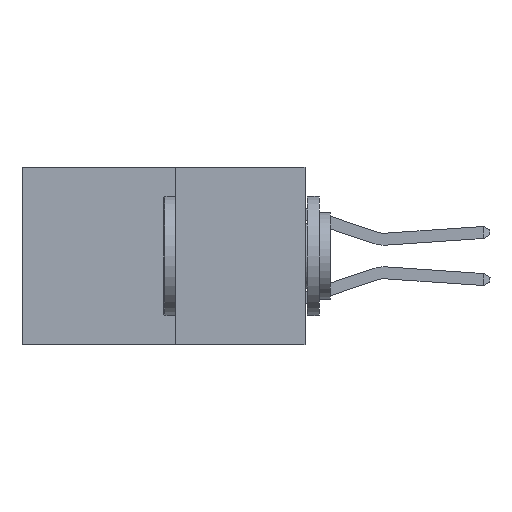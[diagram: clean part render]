
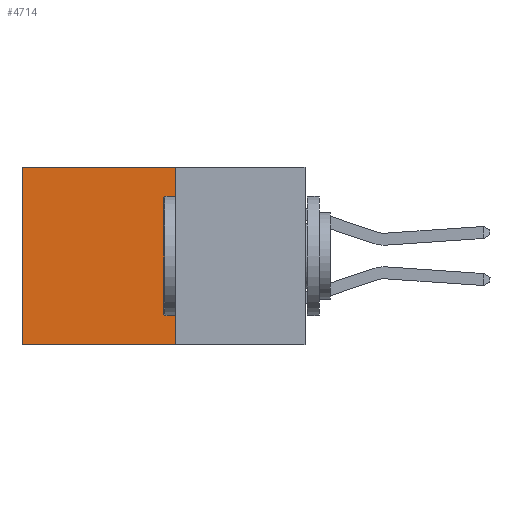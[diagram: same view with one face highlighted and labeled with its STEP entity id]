
A CAD part, left-side view. The second image highlights one B-rep face of the part: STEP entity #4714.
In plain terms, the highlighted planar face has unit normal (-1, 0, 0).
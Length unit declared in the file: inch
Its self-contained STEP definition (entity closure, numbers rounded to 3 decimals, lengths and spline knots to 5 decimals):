
#1151 = VERTEX_POINT ( 'NONE', #15714 ) ;
#1609 = EDGE_CURVE ( 'NONE', #25152, #21305, #25928, .T. ) ;
#1952 = LINE ( 'NONE', #5061, #23638 ) ;
#2919 = EDGE_LOOP ( 'NONE', ( #13480, #12660, #11735, #12608 ) ) ;
#3179 = CARTESIAN_POINT ( 'NONE',  ( 0.277, 0.59, -0.37 ) ) ;
#3272 = VERTEX_POINT ( 'NONE', #8045 ) ;
#3639 = VECTOR ( 'NONE', #25859, 39.37008 ) ;
#4335 = PLANE ( 'NONE',  #7611 ) ;
#4714 = ADVANCED_FACE ( 'NONE', ( #8375 ), #4335, .F. ) ;
#5060 = DIRECTION ( 'NONE',  ( 0., 1., 0. ) ) ;
#5061 = CARTESIAN_POINT ( 'NONE',  ( 0.277, 0.27, -0.37 ) ) ;
#6371 = DIRECTION ( 'NONE',  ( 0., 1., 0. ) ) ;
#7062 = EDGE_CURVE ( 'NONE', #1151, #3272, #1952, .T. ) ;
#7527 = LINE ( 'NONE', #11397, #11865 ) ;
#7611 = AXIS2_PLACEMENT_3D ( 'NONE', #21199, #8630, #23264 ) ;
#8045 = CARTESIAN_POINT ( 'NONE',  ( 0.277, 0.27, -0.37 ) ) ;
#8375 = FACE_OUTER_BOUND ( 'NONE', #2919, .T. ) ;
#8630 = DIRECTION ( 'NONE',  ( 1., 0., 0. ) ) ;
#11397 = CARTESIAN_POINT ( 'NONE',  ( 0.277, 0.27, -0.37 ) ) ;
#11483 = DIRECTION ( 'NONE',  ( 0., 0., -1. ) ) ;
#11735 = ORIENTED_EDGE ( 'NONE', *, *, #7062, .F. ) ;
#11865 = VECTOR ( 'NONE', #5060, 39.37008 ) ;
#12608 = ORIENTED_EDGE ( 'NONE', *, *, #19039, .T. ) ;
#12660 = ORIENTED_EDGE ( 'NONE', *, *, #20539, .F. ) ;
#13480 = ORIENTED_EDGE ( 'NONE', *, *, #1609, .T. ) ;
#15714 = CARTESIAN_POINT ( 'NONE',  ( 0.277, 0.27, 0. ) ) ;
#15874 = CARTESIAN_POINT ( 'NONE',  ( 0.277, 0.59, 0. ) ) ;
#19039 = EDGE_CURVE ( 'NONE', #1151, #25152, #26508, .T. ) ;
#20539 = EDGE_CURVE ( 'NONE', #3272, #21305, #7527, .T. ) ;
#21199 = CARTESIAN_POINT ( 'NONE',  ( 0.277, 0.27, -0.37 ) ) ;
#21305 = VERTEX_POINT ( 'NONE', #3179 ) ;
#23264 = DIRECTION ( 'NONE',  ( 0., 0., -1. ) ) ;
#23465 = CARTESIAN_POINT ( 'NONE',  ( 0.277, 0.59, -0.37 ) ) ;
#23638 = VECTOR ( 'NONE', #11483, 39.37008 ) ;
#25152 = VERTEX_POINT ( 'NONE', #15874 ) ;
#25215 = CARTESIAN_POINT ( 'NONE',  ( 0.277, 0.27, 0. ) ) ;
#25851 = VECTOR ( 'NONE', #6371, 39.37008 ) ;
#25859 = DIRECTION ( 'NONE',  ( 0., 0., -1. ) ) ;
#25928 = LINE ( 'NONE', #23465, #3639 ) ;
#26508 = LINE ( 'NONE', #25215, #25851 ) ;
